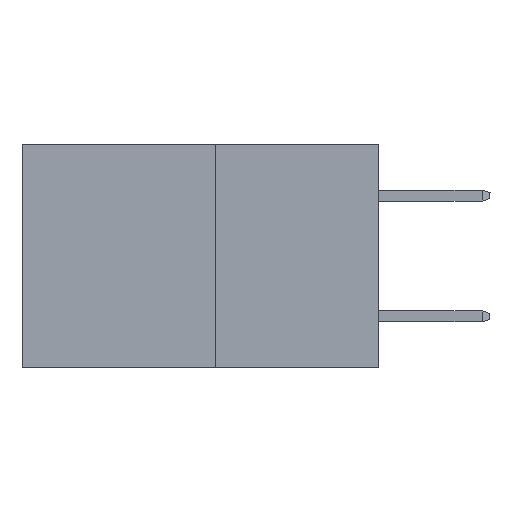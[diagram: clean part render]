
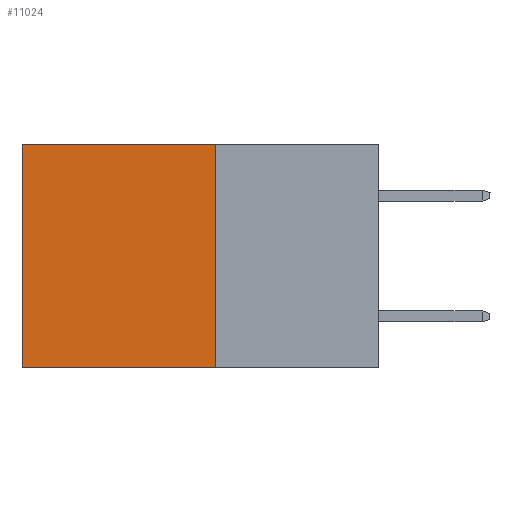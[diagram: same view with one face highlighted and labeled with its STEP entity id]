
A CAD part, left-side view. The second image highlights one B-rep face of the part: STEP entity #11024.
In plain terms, the highlighted planar face has unit normal (-1, 0, 0).
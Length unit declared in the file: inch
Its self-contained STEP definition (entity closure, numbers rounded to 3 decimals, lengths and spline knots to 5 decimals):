
#156 = LINE ( 'NONE', #13742, #18551 ) ;
#2156 = VERTEX_POINT ( 'NONE', #14527 ) ;
#2533 = VECTOR ( 'NONE', #2897, 39.37008 ) ;
#2642 = ORIENTED_EDGE ( 'NONE', *, *, #9105, .F. ) ;
#2802 = ORIENTED_EDGE ( 'NONE', *, *, #18406, .T. ) ;
#2897 = DIRECTION ( 'NONE',  ( 0., 1., 0. ) ) ;
#2929 = CARTESIAN_POINT ( 'NONE',  ( 0.277, 0.27, 0. ) ) ;
#3422 = CARTESIAN_POINT ( 'NONE',  ( 0.277, 0.27, -0.37 ) ) ;
#3872 = EDGE_CURVE ( 'NONE', #15371, #2156, #16658, .T. ) ;
#4867 = PLANE ( 'NONE',  #17709 ) ;
#4932 = DIRECTION ( 'NONE',  ( 0., 0., -1. ) ) ;
#5471 = EDGE_LOOP ( 'NONE', ( #18014, #16579, #2642, #2802 ) ) ;
#7940 = VERTEX_POINT ( 'NONE', #16135 ) ;
#9105 = EDGE_CURVE ( 'NONE', #7940, #18421, #156, .T. ) ;
#10281 = CARTESIAN_POINT ( 'NONE',  ( 0.277, 0.27, -0.37 ) ) ;
#11024 = ADVANCED_FACE ( 'NONE', ( #16785 ), #4867, .F. ) ;
#11753 = DIRECTION ( 'NONE',  ( 0., 1., 0. ) ) ;
#13689 = DIRECTION ( 'NONE',  ( 1., 0., 0. ) ) ;
#13742 = CARTESIAN_POINT ( 'NONE',  ( 0.277, 0.27, -0.37 ) ) ;
#13823 = LINE ( 'NONE', #2929, #2533 ) ;
#14527 = CARTESIAN_POINT ( 'NONE',  ( 0.277, 0.59, -0.37 ) ) ;
#14652 = DIRECTION ( 'NONE',  ( 0., 0., -1. ) ) ;
#15215 = DIRECTION ( 'NONE',  ( 0., 0., -1. ) ) ;
#15371 = VERTEX_POINT ( 'NONE', #18138 ) ;
#15415 = CARTESIAN_POINT ( 'NONE',  ( 0.277, 0.59, -0.37 ) ) ;
#16131 = CARTESIAN_POINT ( 'NONE',  ( 0.277, 0.27, -0.37 ) ) ;
#16135 = CARTESIAN_POINT ( 'NONE',  ( 0.277, 0.27, 0. ) ) ;
#16297 = LINE ( 'NONE', #10281, #18639 ) ;
#16579 = ORIENTED_EDGE ( 'NONE', *, *, #17734, .F. ) ;
#16658 = LINE ( 'NONE', #15415, #17077 ) ;
#16785 = FACE_OUTER_BOUND ( 'NONE', #5471, .T. ) ;
#17077 = VECTOR ( 'NONE', #15215, 39.37008 ) ;
#17709 = AXIS2_PLACEMENT_3D ( 'NONE', #3422, #13689, #4932 ) ;
#17734 = EDGE_CURVE ( 'NONE', #18421, #2156, #16297, .T. ) ;
#18014 = ORIENTED_EDGE ( 'NONE', *, *, #3872, .T. ) ;
#18138 = CARTESIAN_POINT ( 'NONE',  ( 0.277, 0.59, 0. ) ) ;
#18406 = EDGE_CURVE ( 'NONE', #7940, #15371, #13823, .T. ) ;
#18421 = VERTEX_POINT ( 'NONE', #16131 ) ;
#18551 = VECTOR ( 'NONE', #14652, 39.37008 ) ;
#18639 = VECTOR ( 'NONE', #11753, 39.37008 ) ;
